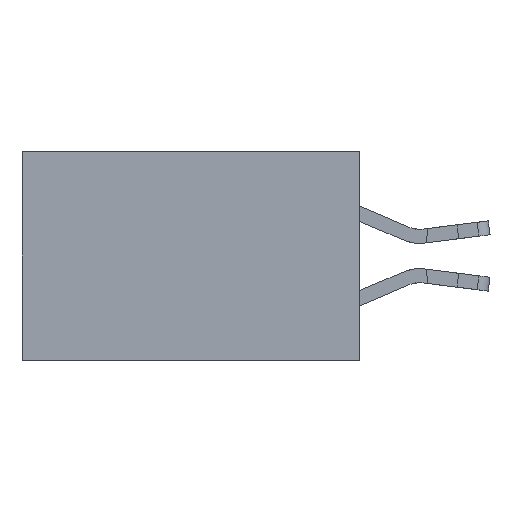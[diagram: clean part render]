
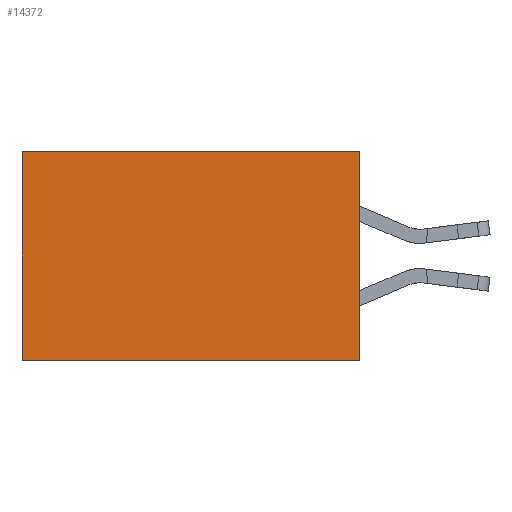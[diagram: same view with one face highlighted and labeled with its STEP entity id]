
A CAD part, left-side view. The second image highlights one B-rep face of the part: STEP entity #14372.
In plain terms, the highlighted planar face has unit normal (-1, 0, 0).
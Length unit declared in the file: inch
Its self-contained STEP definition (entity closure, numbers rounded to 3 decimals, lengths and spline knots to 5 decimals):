
#536 = VECTOR ( 'NONE', #746, 39.37008 ) ;
#746 = DIRECTION ( 'NONE',  ( 0., 1., 0. ) ) ;
#1986 = CARTESIAN_POINT ( 'NONE',  ( 0.2875, 0., -0.37 ) ) ;
#2449 = ORIENTED_EDGE ( 'NONE', *, *, #5312, .T. ) ;
#2793 = EDGE_CURVE ( 'NONE', #17285, #16481, #12740, .T. ) ;
#3706 = EDGE_CURVE ( 'NONE', #12311, #13555, #22807, .T. ) ;
#5259 = DIRECTION ( 'NONE',  ( 0., 0., -1. ) ) ;
#5312 = EDGE_CURVE ( 'NONE', #12311, #17285, #7552, .T. ) ;
#6547 = CARTESIAN_POINT ( 'NONE',  ( 0.2875, 0.6, 0. ) ) ;
#7552 = LINE ( 'NONE', #17064, #536 ) ;
#7610 = CARTESIAN_POINT ( 'NONE',  ( 0.2875, 0.6, 0. ) ) ;
#7917 = CARTESIAN_POINT ( 'NONE',  ( 0.2875, 0., 0. ) ) ;
#7933 = CARTESIAN_POINT ( 'NONE',  ( 0.2875, 0., -0.37 ) ) ;
#8561 = VECTOR ( 'NONE', #22726, 39.37008 ) ;
#8933 = CARTESIAN_POINT ( 'NONE',  ( 0.2875, 0.6, -0.37 ) ) ;
#9940 = ORIENTED_EDGE ( 'NONE', *, *, #3706, .F. ) ;
#10860 = EDGE_LOOP ( 'NONE', ( #15562, #16574, #9940, #2449 ) ) ;
#11629 = DIRECTION ( 'NONE',  ( 1., 0., 0. ) ) ;
#12311 = VERTEX_POINT ( 'NONE', #7917 ) ;
#12383 = AXIS2_PLACEMENT_3D ( 'NONE', #12888, #11629, #18182 ) ;
#12551 = CARTESIAN_POINT ( 'NONE',  ( 0.2875, 0., 0. ) ) ;
#12740 = LINE ( 'NONE', #6547, #8561 ) ;
#12888 = CARTESIAN_POINT ( 'NONE',  ( 0.2875, 0., 0. ) ) ;
#13555 = VERTEX_POINT ( 'NONE', #7933 ) ;
#14372 = ADVANCED_FACE ( 'NONE', ( #18420 ), #18335, .F. ) ;
#15562 = ORIENTED_EDGE ( 'NONE', *, *, #2793, .T. ) ;
#16374 = DIRECTION ( 'NONE',  ( 0., 1., 0. ) ) ;
#16481 = VERTEX_POINT ( 'NONE', #8933 ) ;
#16574 = ORIENTED_EDGE ( 'NONE', *, *, #21567, .F. ) ;
#17064 = CARTESIAN_POINT ( 'NONE',  ( 0.2875, 0., 0. ) ) ;
#17285 = VERTEX_POINT ( 'NONE', #7610 ) ;
#18182 = DIRECTION ( 'NONE',  ( 0., 0., -1. ) ) ;
#18268 = VECTOR ( 'NONE', #5259, 39.37008 ) ;
#18335 = PLANE ( 'NONE',  #12383 ) ;
#18420 = FACE_OUTER_BOUND ( 'NONE', #10860, .T. ) ;
#19082 = VECTOR ( 'NONE', #16374, 39.37008 ) ;
#21567 = EDGE_CURVE ( 'NONE', #13555, #16481, #22729, .T. ) ;
#22726 = DIRECTION ( 'NONE',  ( 0., 0., -1. ) ) ;
#22729 = LINE ( 'NONE', #1986, #19082 ) ;
#22807 = LINE ( 'NONE', #12551, #18268 ) ;
